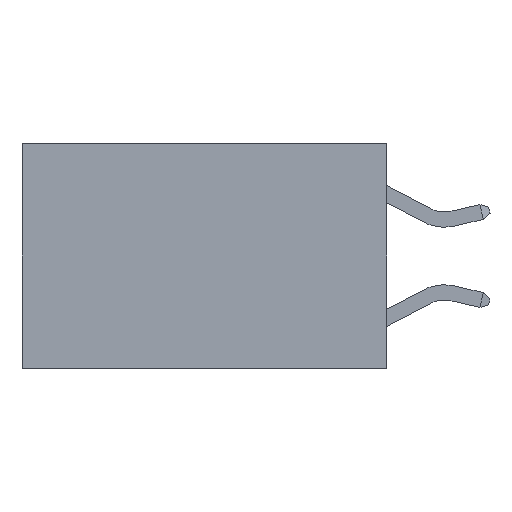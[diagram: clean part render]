
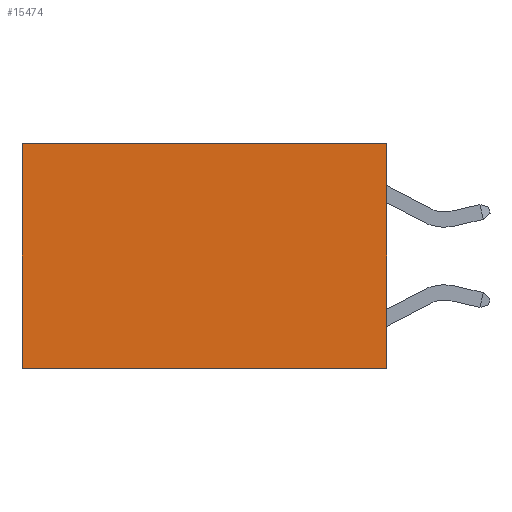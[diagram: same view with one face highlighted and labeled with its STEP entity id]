
A CAD part, left-side view. The second image highlights one B-rep face of the part: STEP entity #15474.
In plain terms, the highlighted planar face has unit normal (-1, 0, 0).
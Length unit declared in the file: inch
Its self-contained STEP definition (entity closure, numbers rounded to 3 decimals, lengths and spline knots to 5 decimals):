
#284 = VERTEX_POINT ( 'NONE', #19201 ) ;
#1232 = EDGE_CURVE ( 'NONE', #284, #21484, #15706, .T. ) ;
#1408 = LINE ( 'NONE', #29361, #6741 ) ;
#1429 = PLANE ( 'NONE',  #3451 ) ;
#1664 = ORIENTED_EDGE ( 'NONE', *, *, #1232, .F. ) ;
#2713 = DIRECTION ( 'NONE',  ( 0., 0., -1. ) ) ;
#3451 = AXIS2_PLACEMENT_3D ( 'NONE', #19698, #26350, #28449 ) ;
#5043 = LINE ( 'NONE', #5232, #23853 ) ;
#5232 = CARTESIAN_POINT ( 'NONE',  ( 0.2625, 0., 0. ) ) ;
#6108 = CARTESIAN_POINT ( 'NONE',  ( 0.2625, 0., 0. ) ) ;
#6226 = VERTEX_POINT ( 'NONE', #6717 ) ;
#6717 = CARTESIAN_POINT ( 'NONE',  ( 0.2625, 0.6, 0. ) ) ;
#6741 = VECTOR ( 'NONE', #2713, 39.37008 ) ;
#7161 = VECTOR ( 'NONE', #26222, 39.37008 ) ;
#7811 = EDGE_LOOP ( 'NONE', ( #24338, #1664, #14018, #27412 ) ) ;
#8126 = EDGE_CURVE ( 'NONE', #6226, #21484, #1408, .T. ) ;
#9267 = VECTOR ( 'NONE', #27163, 39.37008 ) ;
#12334 = EDGE_CURVE ( 'NONE', #21622, #284, #5043, .T. ) ;
#14018 = ORIENTED_EDGE ( 'NONE', *, *, #12334, .F. ) ;
#15474 = ADVANCED_FACE ( 'NONE', ( #21540 ), #1429, .F. ) ;
#15706 = LINE ( 'NONE', #29360, #9267 ) ;
#15709 = LINE ( 'NONE', #6108, #7161 ) ;
#15743 = CARTESIAN_POINT ( 'NONE',  ( 0.2625, 0., 0. ) ) ;
#19201 = CARTESIAN_POINT ( 'NONE',  ( 0.2625, 0., -0.37 ) ) ;
#19498 = EDGE_CURVE ( 'NONE', #21622, #6226, #15709, .T. ) ;
#19698 = CARTESIAN_POINT ( 'NONE',  ( 0.2625, 0., 0. ) ) ;
#21484 = VERTEX_POINT ( 'NONE', #28738 ) ;
#21540 = FACE_OUTER_BOUND ( 'NONE', #7811, .T. ) ;
#21622 = VERTEX_POINT ( 'NONE', #15743 ) ;
#23853 = VECTOR ( 'NONE', #27852, 39.37008 ) ;
#24338 = ORIENTED_EDGE ( 'NONE', *, *, #8126, .T. ) ;
#26222 = DIRECTION ( 'NONE',  ( 0., 1., 0. ) ) ;
#26350 = DIRECTION ( 'NONE',  ( 1., 0., 0. ) ) ;
#27163 = DIRECTION ( 'NONE',  ( 0., 1., 0. ) ) ;
#27412 = ORIENTED_EDGE ( 'NONE', *, *, #19498, .T. ) ;
#27852 = DIRECTION ( 'NONE',  ( 0., 0., -1. ) ) ;
#28449 = DIRECTION ( 'NONE',  ( 0., 0., -1. ) ) ;
#28738 = CARTESIAN_POINT ( 'NONE',  ( 0.2625, 0.6, -0.37 ) ) ;
#29360 = CARTESIAN_POINT ( 'NONE',  ( 0.2625, 0., -0.37 ) ) ;
#29361 = CARTESIAN_POINT ( 'NONE',  ( 0.2625, 0.6, 0. ) ) ;
